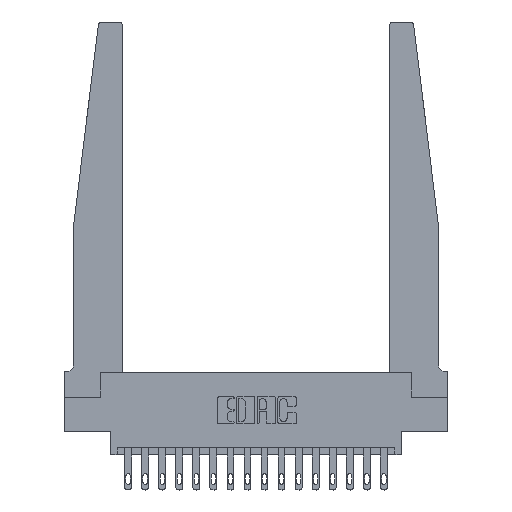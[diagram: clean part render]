
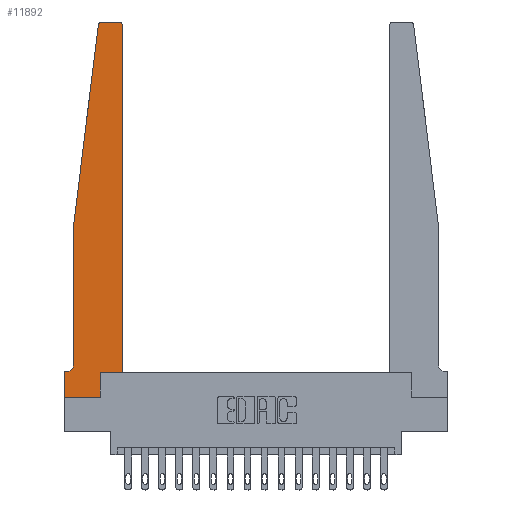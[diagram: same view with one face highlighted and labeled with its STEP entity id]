
A CAD part, top view. The second image highlights one B-rep face of the part: STEP entity #11892.
In plain terms, the highlighted planar face has unit normal (0, 0, 1).
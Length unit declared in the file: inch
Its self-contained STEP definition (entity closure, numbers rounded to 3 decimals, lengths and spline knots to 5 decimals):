
#267 = DIRECTION ( 'NONE',  ( 0., 1., 0. ) ) ;
#474 = CARTESIAN_POINT ( 'NONE',  ( 0.2605, 0.18, 0.37 ) ) ;
#564 = DIRECTION ( 'NONE',  ( 0., 0., 1. ) ) ;
#567 = FACE_OUTER_BOUND ( 'NONE', #7673, .T. ) ;
#687 = CARTESIAN_POINT ( 'NONE',  ( 0.425, 2.72, 0.37 ) ) ;
#746 = VECTOR ( 'NONE', #1061, 39.37008 ) ;
#1061 = DIRECTION ( 'NONE',  ( 1., 0., 0. ) ) ;
#1266 = VERTEX_POINT ( 'NONE', #15473 ) ;
#1399 = VECTOR ( 'NONE', #15696, 39.37008 ) ;
#1703 = ORIENTED_EDGE ( 'NONE', *, *, #12944, .T. ) ;
#1742 = LINE ( 'NONE', #7658, #6868 ) ;
#1940 = CARTESIAN_POINT ( 'NONE',  ( 0.395, 2.72, 0.37 ) ) ;
#2066 = DIRECTION ( 'NONE',  ( 0., 0., -1. ) ) ;
#2600 = CARTESIAN_POINT ( 'NONE',  ( 0., 0., 0.37 ) ) ;
#2792 = VERTEX_POINT ( 'NONE', #16308 ) ;
#3019 = CIRCLE ( 'NONE', #12653, 0.03 ) ;
#3200 = DIRECTION ( 'NONE',  ( 1., 0., 0. ) ) ;
#3210 = ORIENTED_EDGE ( 'NONE', *, *, #15542, .T. ) ;
#3224 = VERTEX_POINT ( 'NONE', #10569 ) ;
#3483 = DIRECTION ( 'NONE',  ( 1., 0., 0. ) ) ;
#3666 = LINE ( 'NONE', #15529, #746 ) ;
#3692 = VECTOR ( 'NONE', #16282, 39.37008 ) ;
#3982 = ORIENTED_EDGE ( 'NONE', *, *, #12100, .T. ) ;
#4241 = ORIENTED_EDGE ( 'NONE', *, *, #13547, .T. ) ;
#4324 = AXIS2_PLACEMENT_3D ( 'NONE', #18389, #2066, #8086 ) ;
#4753 = DIRECTION ( 'NONE',  ( 1., 0., 0. ) ) ;
#5552 = VERTEX_POINT ( 'NONE', #9526 ) ;
#6202 = DIRECTION ( 'NONE',  ( 0., 0., 1. ) ) ;
#6318 = VECTOR ( 'NONE', #19118, 39.37008 ) ;
#6489 = CARTESIAN_POINT ( 'NONE',  ( 0., 0.1875, 0.37 ) ) ;
#6868 = VECTOR ( 'NONE', #267, 39.37008 ) ;
#7098 = EDGE_CURVE ( 'NONE', #10643, #9785, #1742, .T. ) ;
#7159 = LINE ( 'NONE', #2600, #14075 ) ;
#7658 = CARTESIAN_POINT ( 'NONE',  ( 0.425, 0.18, 0.37 ) ) ;
#7671 = PLANE ( 'NONE',  #16890 ) ;
#7673 = EDGE_LOOP ( 'NONE', ( #12965, #3210, #1703, #4241, #8374, #16398, #19026, #11621, #16055, #3982, #14726, #18171 ) ) ;
#7987 = AXIS2_PLACEMENT_3D ( 'NONE', #10893, #564, #3200 ) ;
#8086 = DIRECTION ( 'NONE',  ( -1., 0., 0. ) ) ;
#8113 = CARTESIAN_POINT ( 'NONE',  ( 0., 0., 0.37 ) ) ;
#8229 = LINE ( 'NONE', #8417, #1399 ) ;
#8374 = ORIENTED_EDGE ( 'NONE', *, *, #18184, .T. ) ;
#8417 = CARTESIAN_POINT ( 'NONE',  ( 0.065, 0.1875, 0.37 ) ) ;
#8551 = CARTESIAN_POINT ( 'NONE',  ( 0.27653, 2.75, 0.37 ) ) ;
#8821 = LINE ( 'NONE', #16002, #6318 ) ;
#9526 = CARTESIAN_POINT ( 'NONE',  ( 0.065, 1.25, 0.37 ) ) ;
#9785 = VERTEX_POINT ( 'NONE', #687 ) ;
#10194 = DIRECTION ( 'NONE',  ( 1., 0., 0. ) ) ;
#10267 = CARTESIAN_POINT ( 'NONE',  ( 0.24675, 2.72367, 0.37 ) ) ;
#10378 = CARTESIAN_POINT ( 'NONE',  ( 0.25, 2.75, 0.37 ) ) ;
#10489 = VERTEX_POINT ( 'NONE', #18232 ) ;
#10569 = CARTESIAN_POINT ( 'NONE',  ( 0.065, 0.2375, 0.37 ) ) ;
#10643 = VERTEX_POINT ( 'NONE', #15150 ) ;
#10893 = CARTESIAN_POINT ( 'NONE',  ( 0.27653, 2.72, 0.37 ) ) ;
#11036 = EDGE_CURVE ( 'NONE', #10489, #15625, #8821, .T. ) ;
#11073 = EDGE_CURVE ( 'NONE', #18544, #10489, #7159, .T. ) ;
#11502 = CIRCLE ( 'NONE', #4324, 0.05 ) ;
#11621 = ORIENTED_EDGE ( 'NONE', *, *, #11073, .T. ) ;
#11704 = VECTOR ( 'NONE', #12587, 39.37008 ) ;
#11766 = DIRECTION ( 'NONE',  ( 0., -1., 0. ) ) ;
#11892 = ADVANCED_FACE ( 'NONE', ( #567 ), #7671, .T. ) ;
#12100 = EDGE_CURVE ( 'NONE', #15625, #10643, #3666, .T. ) ;
#12442 = EDGE_CURVE ( 'NONE', #1266, #15324, #8229, .T. ) ;
#12587 = DIRECTION ( 'NONE',  ( 0., -1., 0. ) ) ;
#12653 = AXIS2_PLACEMENT_3D ( 'NONE', #1940, #16610, #4753 ) ;
#12944 = EDGE_CURVE ( 'NONE', #16286, #5552, #14032, .T. ) ;
#12965 = ORIENTED_EDGE ( 'NONE', *, *, #17556, .T. ) ;
#13547 = EDGE_CURVE ( 'NONE', #5552, #3224, #14561, .T. ) ;
#14032 = LINE ( 'NONE', #15394, #14434 ) ;
#14075 = VECTOR ( 'NONE', #10194, 39.37008 ) ;
#14192 = EDGE_CURVE ( 'NONE', #15324, #18544, #16859, .T. ) ;
#14434 = VECTOR ( 'NONE', #18596, 39.37008 ) ;
#14561 = LINE ( 'NONE', #16106, #16617 ) ;
#14726 = ORIENTED_EDGE ( 'NONE', *, *, #7098, .T. ) ;
#15150 = CARTESIAN_POINT ( 'NONE',  ( 0.425, 0.18, 0.37 ) ) ;
#15324 = VERTEX_POINT ( 'NONE', #19143 ) ;
#15394 = CARTESIAN_POINT ( 'NONE',  ( 0.065, 1.25, 0.37 ) ) ;
#15473 = CARTESIAN_POINT ( 'NONE',  ( 0.015, 0.1875, 0.37 ) ) ;
#15497 = EDGE_CURVE ( 'NONE', #9785, #2792, #3019, .T. ) ;
#15529 = CARTESIAN_POINT ( 'NONE',  ( 0.425, 0.18, 0.37 ) ) ;
#15542 = EDGE_CURVE ( 'NONE', #18963, #16286, #16361, .T. ) ;
#15625 = VERTEX_POINT ( 'NONE', #474 ) ;
#15696 = DIRECTION ( 'NONE',  ( -1., 0., 0. ) ) ;
#16002 = CARTESIAN_POINT ( 'NONE',  ( 0.2605, 0.18, 0.37 ) ) ;
#16055 = ORIENTED_EDGE ( 'NONE', *, *, #11036, .T. ) ;
#16106 = CARTESIAN_POINT ( 'NONE',  ( 0.065, 1.25, 0.37 ) ) ;
#16282 = DIRECTION ( 'NONE',  ( -1., 0., 0. ) ) ;
#16286 = VERTEX_POINT ( 'NONE', #10267 ) ;
#16308 = CARTESIAN_POINT ( 'NONE',  ( 0.395, 2.75, 0.37 ) ) ;
#16361 = CIRCLE ( 'NONE', #7987, 0.03 ) ;
#16398 = ORIENTED_EDGE ( 'NONE', *, *, #12442, .T. ) ;
#16610 = DIRECTION ( 'NONE',  ( 0., 0., 1. ) ) ;
#16617 = VECTOR ( 'NONE', #11766, 39.37008 ) ;
#16859 = LINE ( 'NONE', #8113, #11704 ) ;
#16890 = AXIS2_PLACEMENT_3D ( 'NONE', #6489, #6202, #3483 ) ;
#17556 = EDGE_CURVE ( 'NONE', #2792, #18963, #17745, .T. ) ;
#17745 = LINE ( 'NONE', #10378, #3692 ) ;
#18171 = ORIENTED_EDGE ( 'NONE', *, *, #15497, .T. ) ;
#18184 = EDGE_CURVE ( 'NONE', #3224, #1266, #11502, .T. ) ;
#18232 = CARTESIAN_POINT ( 'NONE',  ( 0.2605, 0., 0.37 ) ) ;
#18389 = CARTESIAN_POINT ( 'NONE',  ( 0.015, 0.2375, 0.37 ) ) ;
#18532 = CARTESIAN_POINT ( 'NONE',  ( 0., 0., 0.37 ) ) ;
#18544 = VERTEX_POINT ( 'NONE', #18532 ) ;
#18596 = DIRECTION ( 'NONE',  ( -0.122, -0.992, 0. ) ) ;
#18963 = VERTEX_POINT ( 'NONE', #8551 ) ;
#19026 = ORIENTED_EDGE ( 'NONE', *, *, #14192, .T. ) ;
#19118 = DIRECTION ( 'NONE',  ( 0., 1., 0. ) ) ;
#19143 = CARTESIAN_POINT ( 'NONE',  ( 0., 0.1875, 0.37 ) ) ;
